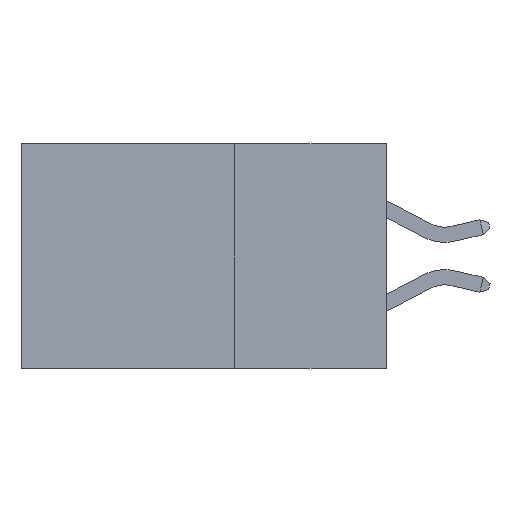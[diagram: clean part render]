
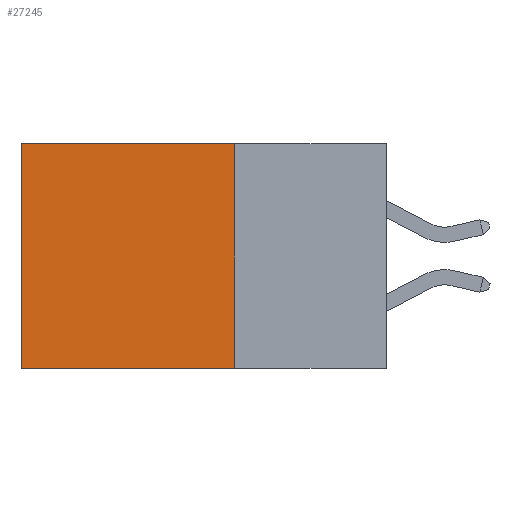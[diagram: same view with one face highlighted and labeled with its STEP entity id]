
A CAD part, left-side view. The second image highlights one B-rep face of the part: STEP entity #27245.
In plain terms, the highlighted planar face has unit normal (-1, 0, 0).
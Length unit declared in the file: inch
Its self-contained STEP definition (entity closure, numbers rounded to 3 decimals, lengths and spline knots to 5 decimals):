
#518 = CARTESIAN_POINT ( 'NONE',  ( 0.2615, 0.25, -0.37 ) ) ;
#546 = ORIENTED_EDGE ( 'NONE', *, *, #2252, .T. ) ;
#1508 = VECTOR ( 'NONE', #13457, 39.37008 ) ;
#1619 = VECTOR ( 'NONE', #21734, 39.37008 ) ;
#1880 = DIRECTION ( 'NONE',  ( 1., 0., 0. ) ) ;
#2252 = EDGE_CURVE ( 'NONE', #11784, #27297, #17479, .T. ) ;
#3824 = LINE ( 'NONE', #18894, #20315 ) ;
#3851 = DIRECTION ( 'NONE',  ( 0., 1., 0. ) ) ;
#3994 = CARTESIAN_POINT ( 'NONE',  ( 0.2615, 0.25, -0.37 ) ) ;
#4065 = EDGE_CURVE ( 'NONE', #21471, #27297, #18045, .T. ) ;
#4231 = ORIENTED_EDGE ( 'NONE', *, *, #4065, .F. ) ;
#5253 = EDGE_LOOP ( 'NONE', ( #546, #4231, #26915, #23557 ) ) ;
#5634 = VERTEX_POINT ( 'NONE', #17267 ) ;
#6651 = EDGE_CURVE ( 'NONE', #5634, #21471, #17266, .T. ) ;
#7403 = FACE_OUTER_BOUND ( 'NONE', #5253, .T. ) ;
#9675 = CARTESIAN_POINT ( 'NONE',  ( 0.2615, 0.6, 0. ) ) ;
#11784 = VERTEX_POINT ( 'NONE', #9675 ) ;
#11910 = DIRECTION ( 'NONE',  ( 0., 0., -1. ) ) ;
#13457 = DIRECTION ( 'NONE',  ( 0., 1., 0. ) ) ;
#13517 = CARTESIAN_POINT ( 'NONE',  ( 0.2615, 0.25, -0.37 ) ) ;
#14991 = CARTESIAN_POINT ( 'NONE',  ( 0.2615, 0.6, -0.37 ) ) ;
#16966 = DIRECTION ( 'NONE',  ( 0., 0., -1. ) ) ;
#17266 = LINE ( 'NONE', #24718, #22964 ) ;
#17267 = CARTESIAN_POINT ( 'NONE',  ( 0.2615, 0.25, 0. ) ) ;
#17479 = LINE ( 'NONE', #18738, #1619 ) ;
#18008 = EDGE_CURVE ( 'NONE', #5634, #11784, #3824, .T. ) ;
#18045 = LINE ( 'NONE', #13517, #1508 ) ;
#18738 = CARTESIAN_POINT ( 'NONE',  ( 0.2615, 0.6, -0.37 ) ) ;
#18894 = CARTESIAN_POINT ( 'NONE',  ( 0.2615, 0.25, 0. ) ) ;
#20315 = VECTOR ( 'NONE', #3851, 39.37008 ) ;
#21471 = VERTEX_POINT ( 'NONE', #518 ) ;
#21734 = DIRECTION ( 'NONE',  ( 0., 0., -1. ) ) ;
#22964 = VECTOR ( 'NONE', #11910, 39.37008 ) ;
#23557 = ORIENTED_EDGE ( 'NONE', *, *, #18008, .T. ) ;
#24718 = CARTESIAN_POINT ( 'NONE',  ( 0.2615, 0.25, -0.37 ) ) ;
#25481 = PLANE ( 'NONE',  #26291 ) ;
#26291 = AXIS2_PLACEMENT_3D ( 'NONE', #3994, #1880, #16966 ) ;
#26915 = ORIENTED_EDGE ( 'NONE', *, *, #6651, .F. ) ;
#27245 = ADVANCED_FACE ( 'NONE', ( #7403 ), #25481, .F. ) ;
#27297 = VERTEX_POINT ( 'NONE', #14991 ) ;
